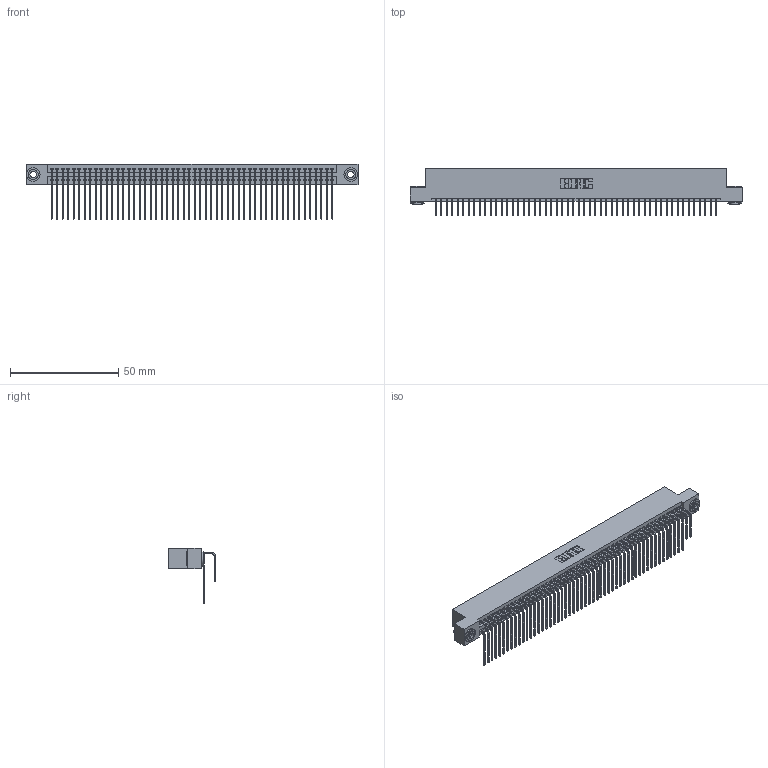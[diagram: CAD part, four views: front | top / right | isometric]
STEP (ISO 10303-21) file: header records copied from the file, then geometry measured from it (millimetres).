
FILE_DESCRIPTION (( 'STEP AP203' ), '1' );
FILE_NAME ('345-104-558-203.STEP', '2019-11-03T13:05:32', ( '' ), ( '' ), 'SwSTEP 2.0', 'SolidWorks 2016', '' );
FILE_SCHEMA (( 'CONFIG_CONTROL_DESIGN' ));
Length unit declared in the file: inch
Products named in the file (5): 345 Part_Flush Mounting Lugs - 0.156 Dia-TH; 345-292-001_558 Tail - 2; 345-292-001_558 559 Tail - 1; 345-250-002_345-250-002-102; 345-104-558-203
Assembly tree (107 placements, depth 2):
  345-104-558-203
    345 Part_Flush Mounting Lugs - 0.156 Dia-TH
    345-292-001_558 559 Tail - 1  x52
    345-292-001_558 Tail - 2  x52
    345-250-002_345-250-002-102  x2
Bounding box: 153.29 x 21.83 x 25.53 mm (x, y, z)
Volume: 15602.8 mm3; surface area: 26283.3 mm2
Topology: 107 solids, 107 shells, 5572 faces, 16537 edges, 10882 vertices
Faces by surface type: plane 3730, cylinder 1834, cone 8
Entity records: 41756 total; most frequent: CARTESIAN_POINT 7010, ORIENTED_EDGE 6886, DIRECTION 6173, EDGE_CURVE 3443, LINE 3039, VECTOR 3039, VERTEX_POINT 2290, AXIS2_PLACEMENT_3D 1567
